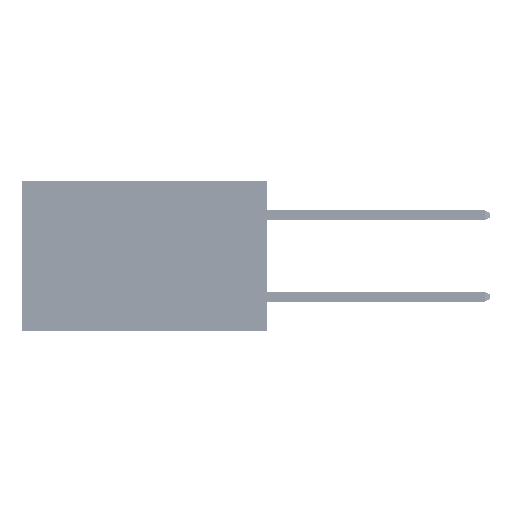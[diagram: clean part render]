
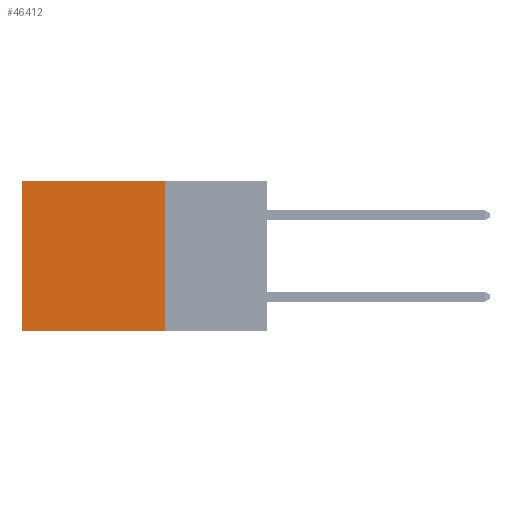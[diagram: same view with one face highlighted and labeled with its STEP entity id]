
A CAD part, left-side view. The second image highlights one B-rep face of the part: STEP entity #46412.
In plain terms, the highlighted planar face has unit normal (-1, 0, 0).
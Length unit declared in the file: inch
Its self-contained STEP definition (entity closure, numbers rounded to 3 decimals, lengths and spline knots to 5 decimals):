
#1217 = CARTESIAN_POINT ( 'NONE',  ( 0.2875, 0.6, 0. ) ) ;
#1782 = PLANE ( 'NONE',  #49310 ) ;
#5097 = LINE ( 'NONE', #1217, #19817 ) ;
#5917 = DIRECTION ( 'NONE',  ( 1., 0., 0. ) ) ;
#7921 = ORIENTED_EDGE ( 'NONE', *, *, #23251, .F. ) ;
#8478 = VERTEX_POINT ( 'NONE', #16453 ) ;
#9240 = EDGE_CURVE ( 'NONE', #26397, #32704, #10428, .T. ) ;
#9697 = ORIENTED_EDGE ( 'NONE', *, *, #17458, .T. ) ;
#10428 = LINE ( 'NONE', #26154, #46181 ) ;
#10589 = CARTESIAN_POINT ( 'NONE',  ( 0.2875, 0.6, -0.37 ) ) ;
#12753 = DIRECTION ( 'NONE',  ( 0., 1., 0. ) ) ;
#16453 = CARTESIAN_POINT ( 'NONE',  ( 0.2875, 0.6, 0. ) ) ;
#16784 = DIRECTION ( 'NONE',  ( 0., 0., -1. ) ) ;
#16962 = DIRECTION ( 'NONE',  ( 0., 0., -1. ) ) ;
#17458 = EDGE_CURVE ( 'NONE', #8478, #34132, #5097, .T. ) ;
#17534 = CARTESIAN_POINT ( 'NONE',  ( 0.2875, 0.25, 0. ) ) ;
#19817 = VECTOR ( 'NONE', #16962, 39.37008 ) ;
#20074 = VECTOR ( 'NONE', #41020, 39.37008 ) ;
#21613 = CARTESIAN_POINT ( 'NONE',  ( 0.2875, 0.25, -0.37 ) ) ;
#23251 = EDGE_CURVE ( 'NONE', #32704, #34132, #25806, .T. ) ;
#25806 = LINE ( 'NONE', #37896, #20074 ) ;
#26154 = CARTESIAN_POINT ( 'NONE',  ( 0.2875, 0.25, 0. ) ) ;
#26397 = VERTEX_POINT ( 'NONE', #44408 ) ;
#30019 = EDGE_LOOP ( 'NONE', ( #9697, #7921, #47450, #48718 ) ) ;
#30273 = DIRECTION ( 'NONE',  ( 0., 0., -1. ) ) ;
#32704 = VERTEX_POINT ( 'NONE', #21613 ) ;
#32831 = LINE ( 'NONE', #49106, #42537 ) ;
#34132 = VERTEX_POINT ( 'NONE', #10589 ) ;
#37106 = FACE_OUTER_BOUND ( 'NONE', #30019, .T. ) ;
#37896 = CARTESIAN_POINT ( 'NONE',  ( 0.2875, 0.25, -0.37 ) ) ;
#41020 = DIRECTION ( 'NONE',  ( 0., 1., 0. ) ) ;
#42537 = VECTOR ( 'NONE', #12753, 39.37008 ) ;
#43732 = EDGE_CURVE ( 'NONE', #26397, #8478, #32831, .T. ) ;
#44408 = CARTESIAN_POINT ( 'NONE',  ( 0.2875, 0.25, 0. ) ) ;
#46181 = VECTOR ( 'NONE', #30273, 39.37008 ) ;
#46412 = ADVANCED_FACE ( 'NONE', ( #37106 ), #1782, .F. ) ;
#47450 = ORIENTED_EDGE ( 'NONE', *, *, #9240, .F. ) ;
#48718 = ORIENTED_EDGE ( 'NONE', *, *, #43732, .T. ) ;
#49106 = CARTESIAN_POINT ( 'NONE',  ( 0.2875, 0.25, 0. ) ) ;
#49310 = AXIS2_PLACEMENT_3D ( 'NONE', #17534, #5917, #16784 ) ;
